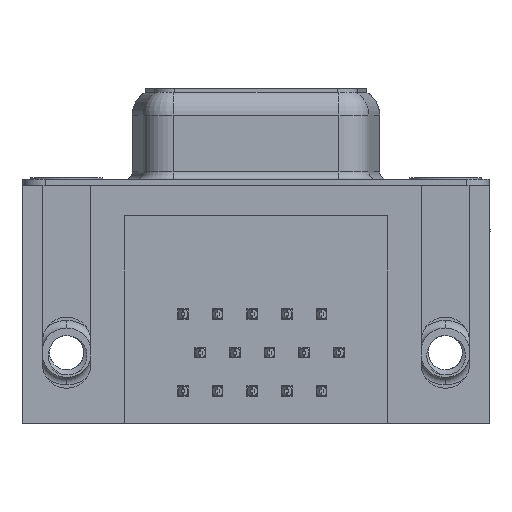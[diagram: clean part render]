
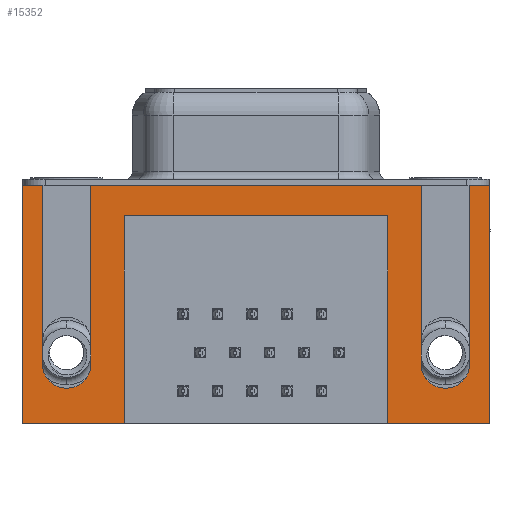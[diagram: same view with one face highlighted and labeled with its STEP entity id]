
A CAD part, front view. The second image highlights one B-rep face of the part: STEP entity #15352.
In plain terms, the highlighted planar face has unit normal (0, -1, 0).
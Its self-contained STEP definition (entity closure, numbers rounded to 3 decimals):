
#15 = ORIENTED_EDGE ( 'NONE', *, *, #18084, .F. ) ;
#154 = CARTESIAN_POINT ( 'NONE',  ( 3.79, -6.275, -15.7 ) ) ;
#279 = CARTESIAN_POINT ( 'NONE',  ( 24.99, -6.275, -11.78 ) ) ;
#621 = DIRECTION ( 'NONE',  ( 0., 0., -1. ) ) ;
#756 = DIRECTION ( 'NONE',  ( 1., 0., 0. ) ) ;
#980 = DIRECTION ( 'NONE',  ( 0., 0., 1. ) ) ;
#1129 = VECTOR ( 'NONE', #22466, 1000. ) ;
#1546 = LINE ( 'NONE', #12140, #9074 ) ;
#1576 = LINE ( 'NONE', #28877, #17625 ) ;
#2874 = LINE ( 'NONE', #31692, #17175 ) ;
#2879 = ORIENTED_EDGE ( 'NONE', *, *, #33795, .F. ) ;
#3067 = DIRECTION ( 'NONE',  ( -1., 0., 0. ) ) ;
#3110 = AXIS2_PLACEMENT_3D ( 'NONE', #279, #20223, #3067 ) ;
#4346 = CARTESIAN_POINT ( 'NONE',  ( 3.79, -6.275, -2. ) ) ;
#4515 = DIRECTION ( 'NONE',  ( 0., 0., 1. ) ) ;
#4749 = CARTESIAN_POINT ( 'NONE',  ( -2.91, -6.275, 0. ) ) ;
#5031 = LINE ( 'NONE', #17420, #12632 ) ;
#5060 = ORIENTED_EDGE ( 'NONE', *, *, #18656, .F. ) ;
#5496 = VERTEX_POINT ( 'NONE', #22982 ) ;
#6499 = FACE_OUTER_BOUND ( 'NONE', #28773, .T. ) ;
#6904 = VERTEX_POINT ( 'NONE', #21371 ) ;
#7290 = DIRECTION ( 'NONE',  ( 0., -1., 0. ) ) ;
#7993 = EDGE_CURVE ( 'NONE', #18809, #16530, #15746, .T. ) ;
#8645 = LINE ( 'NONE', #10939, #1129 ) ;
#9029 = ORIENTED_EDGE ( 'NONE', *, *, #18594, .F. ) ;
#9052 = VECTOR ( 'NONE', #756, 1000. ) ;
#9074 = VECTOR ( 'NONE', #34805, 1000. ) ;
#9711 = DIRECTION ( 'NONE',  ( -1., 0., 0. ) ) ;
#10044 = LINE ( 'NONE', #16877, #16769 ) ;
#10511 = VECTOR ( 'NONE', #980, 1000. ) ;
#10595 = CARTESIAN_POINT ( 'NONE',  ( 23.39, -6.275, -11.78 ) ) ;
#10856 = CARTESIAN_POINT ( 'NONE',  ( 23.39, -6.275, 0. ) ) ;
#10888 = VECTOR ( 'NONE', #621, 1000. ) ;
#10939 = CARTESIAN_POINT ( 'NONE',  ( -1.6, -6.275, 0. ) ) ;
#11334 = CARTESIAN_POINT ( 'NONE',  ( 26.59, -6.275, 0. ) ) ;
#12088 = ORIENTED_EDGE ( 'NONE', *, *, #18814, .F. ) ;
#12140 = CARTESIAN_POINT ( 'NONE',  ( 3.79, -6.275, -2. ) ) ;
#12632 = VECTOR ( 'NONE', #26028, 1000. ) ;
#12671 = VECTOR ( 'NONE', #28398, 1000. ) ;
#12987 = ORIENTED_EDGE ( 'NONE', *, *, #7993, .F. ) ;
#12992 = CARTESIAN_POINT ( 'NONE',  ( 0., -6.275, -11.78 ) ) ;
#13133 = DIRECTION ( 'NONE',  ( 1., 0., 0. ) ) ;
#13314 = VERTEX_POINT ( 'NONE', #30635 ) ;
#13952 = VECTOR ( 'NONE', #20639, 1000. ) ;
#14145 = ORIENTED_EDGE ( 'NONE', *, *, #34999, .F. ) ;
#14487 = CARTESIAN_POINT ( 'NONE',  ( 26.59, -6.275, 0. ) ) ;
#14510 = DIRECTION ( 'NONE',  ( 0., 0., -1. ) ) ;
#14573 = DIRECTION ( 'NONE',  ( 1., 0., 0. ) ) ;
#14854 = ORIENTED_EDGE ( 'NONE', *, *, #17101, .F. ) ;
#15352 = ADVANCED_FACE ( 'NONE', ( #6499 ), #24438, .T. ) ;
#15378 = LINE ( 'NONE', #4749, #36328 ) ;
#15746 = LINE ( 'NONE', #17788, #9052 ) ;
#15870 = DIRECTION ( 'NONE',  ( 1., 0., 0. ) ) ;
#16530 = VERTEX_POINT ( 'NONE', #18181 ) ;
#16617 = CARTESIAN_POINT ( 'NONE',  ( 21.2, -6.275, -2. ) ) ;
#16769 = VECTOR ( 'NONE', #33906, 1000. ) ;
#16857 = AXIS2_PLACEMENT_3D ( 'NONE', #32849, #7290, #27302 ) ;
#16877 = CARTESIAN_POINT ( 'NONE',  ( 27.9, -6.275, -2.5 ) ) ;
#17101 = EDGE_CURVE ( 'NONE', #5496, #18809, #25725, .T. ) ;
#17175 = VECTOR ( 'NONE', #14573, 1000. ) ;
#17420 = CARTESIAN_POINT ( 'NONE',  ( 27.9, -6.275, -15.7 ) ) ;
#17451 = EDGE_CURVE ( 'NONE', #36433, #35425, #10044, .T. ) ;
#17625 = VECTOR ( 'NONE', #14510, 1000. ) ;
#17724 = CARTESIAN_POINT ( 'NONE',  ( -2.91, -6.275, 0. ) ) ;
#17746 = CARTESIAN_POINT ( 'NONE',  ( 27.9, -6.275, 0. ) ) ;
#17788 = CARTESIAN_POINT ( 'NONE',  ( -2.91, -6.275, 0. ) ) ;
#17927 = EDGE_CURVE ( 'NONE', #34342, #18582, #21233, .T. ) ;
#17982 = EDGE_CURVE ( 'NONE', #35812, #34342, #27014, .T. ) ;
#18084 = EDGE_CURVE ( 'NONE', #26038, #35812, #1576, .T. ) ;
#18181 = CARTESIAN_POINT ( 'NONE',  ( -1.6, -6.275, 0. ) ) ;
#18302 = EDGE_CURVE ( 'NONE', #33897, #13314, #18965, .T. ) ;
#18423 = EDGE_CURVE ( 'NONE', #16530, #6904, #8645, .T. ) ;
#18582 = VERTEX_POINT ( 'NONE', #14487 ) ;
#18594 = EDGE_CURVE ( 'NONE', #26520, #5496, #5031, .T. ) ;
#18656 = EDGE_CURVE ( 'NONE', #35007, #26520, #34490, .T. ) ;
#18709 = EDGE_CURVE ( 'NONE', #20141, #35007, #1546, .T. ) ;
#18809 = VERTEX_POINT ( 'NONE', #17724 ) ;
#18814 = EDGE_CURVE ( 'NONE', #23902, #20141, #21637, .T. ) ;
#18925 = LINE ( 'NONE', #26843, #29132 ) ;
#18933 = EDGE_CURVE ( 'NONE', #36433, #23902, #18925, .T. ) ;
#18965 = LINE ( 'NONE', #27307, #33165 ) ;
#20141 = VERTEX_POINT ( 'NONE', #16617 ) ;
#20223 = DIRECTION ( 'NONE',  ( 0., -1., 0. ) ) ;
#20498 = ORIENTED_EDGE ( 'NONE', *, *, #18302, .F. ) ;
#20639 = DIRECTION ( 'NONE',  ( 0., 0., 1. ) ) ;
#21233 = LINE ( 'NONE', #11334, #12671 ) ;
#21371 = CARTESIAN_POINT ( 'NONE',  ( -1.6, -6.275, -11.78 ) ) ;
#21481 = ORIENTED_EDGE ( 'NONE', *, *, #18709, .F. ) ;
#21637 = LINE ( 'NONE', #29036, #13952 ) ;
#22466 = DIRECTION ( 'NONE',  ( 0., 0., -1. ) ) ;
#22982 = CARTESIAN_POINT ( 'NONE',  ( -2.91, -6.275, -15.7 ) ) ;
#23318 = CARTESIAN_POINT ( 'NONE',  ( 3.79, -6.275, -2. ) ) ;
#23902 = VERTEX_POINT ( 'NONE', #24617 ) ;
#23958 = CARTESIAN_POINT ( 'NONE',  ( 26.59, -6.275, -11.78 ) ) ;
#24438 = PLANE ( 'NONE',  #16857 ) ;
#24617 = CARTESIAN_POINT ( 'NONE',  ( 21.2, -6.275, -15.7 ) ) ;
#25545 = CARTESIAN_POINT ( 'NONE',  ( 27.9, -6.275, -15.7 ) ) ;
#25613 = CIRCLE ( 'NONE', #32387, 1.6 ) ;
#25725 = LINE ( 'NONE', #32191, #10511 ) ;
#26028 = DIRECTION ( 'NONE',  ( -1., 0., 0. ) ) ;
#26038 = VERTEX_POINT ( 'NONE', #10856 ) ;
#26238 = CARTESIAN_POINT ( 'NONE',  ( 1.6, -6.275, -11.78 ) ) ;
#26520 = VERTEX_POINT ( 'NONE', #154 ) ;
#26843 = CARTESIAN_POINT ( 'NONE',  ( 27.9, -6.275, -15.7 ) ) ;
#27014 = CIRCLE ( 'NONE', #3110, 1.6 ) ;
#27302 = DIRECTION ( 'NONE',  ( 0., 0., -1. ) ) ;
#27307 = CARTESIAN_POINT ( 'NONE',  ( 1.6, -6.275, 0. ) ) ;
#28223 = ORIENTED_EDGE ( 'NONE', *, *, #17927, .F. ) ;
#28398 = DIRECTION ( 'NONE',  ( 0., 0., 1. ) ) ;
#28773 = EDGE_LOOP ( 'NONE', ( #28223, #35360, #15, #29045, #20498, #14145, #32206, #12987, #14854, #9029, #5060, #21481, #12088, #34466, #30416, #2879 ) ) ;
#28877 = CARTESIAN_POINT ( 'NONE',  ( 23.39, -6.275, 0. ) ) ;
#29036 = CARTESIAN_POINT ( 'NONE',  ( 21.2, -6.275, -2. ) ) ;
#29045 = ORIENTED_EDGE ( 'NONE', *, *, #33201, .F. ) ;
#29132 = VECTOR ( 'NONE', #9711, 1000. ) ;
#30416 = ORIENTED_EDGE ( 'NONE', *, *, #17451, .T. ) ;
#30635 = CARTESIAN_POINT ( 'NONE',  ( 1.6, -6.275, 0. ) ) ;
#31692 = CARTESIAN_POINT ( 'NONE',  ( -2.91, -6.275, 0. ) ) ;
#32191 = CARTESIAN_POINT ( 'NONE',  ( -2.91, -6.275, -2.5 ) ) ;
#32206 = ORIENTED_EDGE ( 'NONE', *, *, #18423, .F. ) ;
#32387 = AXIS2_PLACEMENT_3D ( 'NONE', #12992, #32943, #15870 ) ;
#32849 = CARTESIAN_POINT ( 'NONE',  ( -2.91, -6.275, -2.5 ) ) ;
#32943 = DIRECTION ( 'NONE',  ( 0., -1., 0. ) ) ;
#33165 = VECTOR ( 'NONE', #4515, 1000. ) ;
#33201 = EDGE_CURVE ( 'NONE', #13314, #26038, #15378, .T. ) ;
#33795 = EDGE_CURVE ( 'NONE', #18582, #35425, #2874, .T. ) ;
#33897 = VERTEX_POINT ( 'NONE', #26238 ) ;
#33906 = DIRECTION ( 'NONE',  ( 0., 0., 1. ) ) ;
#34342 = VERTEX_POINT ( 'NONE', #23958 ) ;
#34466 = ORIENTED_EDGE ( 'NONE', *, *, #18933, .F. ) ;
#34490 = LINE ( 'NONE', #23318, #10888 ) ;
#34805 = DIRECTION ( 'NONE',  ( -1., 0., 0. ) ) ;
#34999 = EDGE_CURVE ( 'NONE', #6904, #33897, #25613, .T. ) ;
#35007 = VERTEX_POINT ( 'NONE', #4346 ) ;
#35360 = ORIENTED_EDGE ( 'NONE', *, *, #17982, .F. ) ;
#35425 = VERTEX_POINT ( 'NONE', #17746 ) ;
#35812 = VERTEX_POINT ( 'NONE', #10595 ) ;
#36328 = VECTOR ( 'NONE', #13133, 1000. ) ;
#36433 = VERTEX_POINT ( 'NONE', #25545 ) ;
